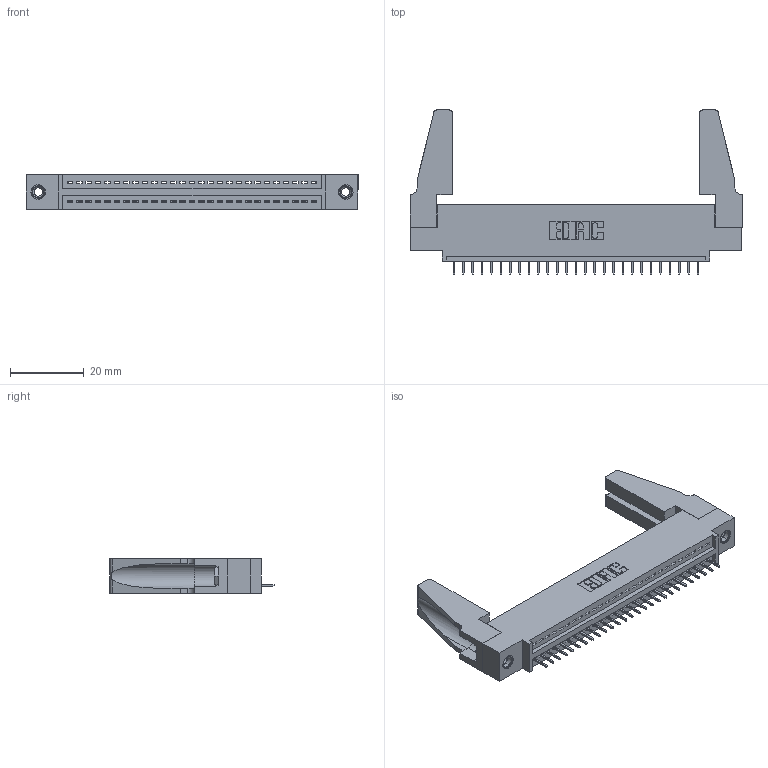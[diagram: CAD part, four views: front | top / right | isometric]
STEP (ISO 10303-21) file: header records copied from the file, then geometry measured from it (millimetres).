
FILE_DESCRIPTION (( 'STEP AP203' ), '1' );
FILE_NAME ('395-027-525-488.STEP', '2020-09-23T16:57:40', ( '' ), ( '' ), 'SwSTEP 2.0', 'SolidWorks 2020', '' );
FILE_SCHEMA (( 'CONFIG_CONTROL_DESIGN' ));
Length unit declared in the file: inch
Products named in the file (5): 345-250-001_345-250-001-102; 345-292-001_345-293-125; 395-027-525-488; 345-220-078_345-220-088; 345 Part_0.110 Offset - 0.156 Dia-TH
Assembly tree (32 placements, depth 2):
  395-027-525-488
    345 Part_0.110 Offset - 0.156 Dia-TH
    345-292-001_345-293-125  x27
    345-250-001_345-250-001-102  x2
    345-220-078_345-220-088  x2
Bounding box: 89.81 x 44.37 x 9.4 mm (x, y, z)
Volume: 11476.7 mm3; surface area: 13568.9 mm2
Topology: 32 solids, 32 shells, 1928 faces, 5527 edges, 3566 vertices
Faces by surface type: plane 1398, cylinder 514, cone 12, torus 4
Entity records: 24694 total; most frequent: CARTESIAN_POINT 4267, ORIENTED_EDGE 4188, DIRECTION 3756, EDGE_CURVE 2094, VECTOR 1816, LINE 1816, VERTEX_POINT 1386, AXIS2_PLACEMENT_3D 970
